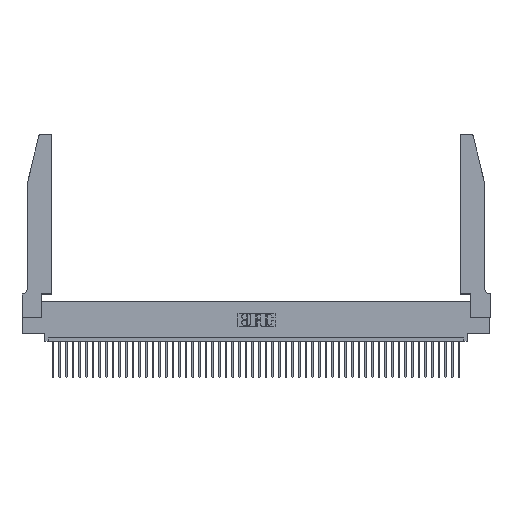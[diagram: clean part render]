
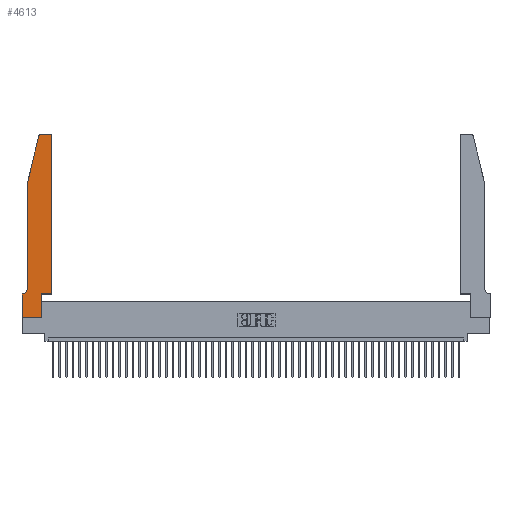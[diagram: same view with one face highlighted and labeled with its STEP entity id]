
A CAD part, top view. The second image highlights one B-rep face of the part: STEP entity #4613.
In plain terms, the highlighted planar face has unit normal (0, 0, 1).
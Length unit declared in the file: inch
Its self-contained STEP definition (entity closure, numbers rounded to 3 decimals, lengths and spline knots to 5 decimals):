
#395 = VERTEX_POINT ( 'NONE', #43126 ) ;
#557 = ORIENTED_EDGE ( 'NONE', *, *, #23836, .T. ) ;
#983 = DIRECTION ( 'NONE',  ( 0., -1., 0. ) ) ;
#1097 = CARTESIAN_POINT ( 'NONE',  ( 0.0755, 0.42, 0.37 ) ) ;
#1267 = CARTESIAN_POINT ( 'NONE',  ( 0.284, 2.72, 0.37 ) ) ;
#1682 = ORIENTED_EDGE ( 'NONE', *, *, #11763, .T. ) ;
#2705 = LINE ( 'NONE', #34800, #46370 ) ;
#3208 = CARTESIAN_POINT ( 'NONE',  ( 0.0755, 2., 0.37 ) ) ;
#3224 = ORIENTED_EDGE ( 'NONE', *, *, #18024, .T. ) ;
#3240 = VERTEX_POINT ( 'NONE', #15658 ) ;
#3483 = CIRCLE ( 'NONE', #43218, 0.03 ) ;
#4543 = LINE ( 'NONE', #46883, #14045 ) ;
#4613 = ADVANCED_FACE ( 'NONE', ( #15782 ), #11750, .T. ) ;
#5359 = VERTEX_POINT ( 'NONE', #21360 ) ;
#5878 = DIRECTION ( 'NONE',  ( -0.239, -0.971, 0. ) ) ;
#5913 = CARTESIAN_POINT ( 'NONE',  ( 0., 0., 0.37 ) ) ;
#6184 = ORIENTED_EDGE ( 'NONE', *, *, #33847, .T. ) ;
#8842 = DIRECTION ( 'NONE',  ( 0., 1., 0. ) ) ;
#9251 = VERTEX_POINT ( 'NONE', #22373 ) ;
#9542 = VECTOR ( 'NONE', #29559, 39.37008 ) ;
#10167 = CARTESIAN_POINT ( 'NONE',  ( 0.0755, 2., 0.37 ) ) ;
#10776 = LINE ( 'NONE', #3208, #9542 ) ;
#11305 = ORIENTED_EDGE ( 'NONE', *, *, #46150, .T. ) ;
#11508 = VERTEX_POINT ( 'NONE', #1097 ) ;
#11750 = PLANE ( 'NONE',  #26635 ) ;
#11763 = EDGE_CURVE ( 'NONE', #17399, #24518, #3483, .T. ) ;
#12138 = ORIENTED_EDGE ( 'NONE', *, *, #13380, .T. ) ;
#12167 = DIRECTION ( 'NONE',  ( -1., 0., 0. ) ) ;
#12723 = VECTOR ( 'NONE', #5878, 39.37008 ) ;
#13380 = EDGE_CURVE ( 'NONE', #32397, #20849, #27481, .T. ) ;
#14045 = VECTOR ( 'NONE', #28001, 39.37008 ) ;
#15224 = VECTOR ( 'NONE', #983, 39.37008 ) ;
#15658 = CARTESIAN_POINT ( 'NONE',  ( 0.2865, 0.35, 0.37 ) ) ;
#15782 = FACE_OUTER_BOUND ( 'NONE', #29788, .T. ) ;
#15824 = ORIENTED_EDGE ( 'NONE', *, *, #44892, .T. ) ;
#15880 = EDGE_CURVE ( 'NONE', #45761, #5359, #39100, .T. ) ;
#15963 = ORIENTED_EDGE ( 'NONE', *, *, #36698, .T. ) ;
#17399 = VERTEX_POINT ( 'NONE', #23423 ) ;
#17493 = EDGE_CURVE ( 'NONE', #3240, #395, #4543, .T. ) ;
#17901 = ORIENTED_EDGE ( 'NONE', *, *, #27004, .T. ) ;
#18024 = EDGE_CURVE ( 'NONE', #11508, #27484, #38205, .T. ) ;
#19718 = DIRECTION ( 'NONE',  ( 1., 0., 0. ) ) ;
#20698 = CARTESIAN_POINT ( 'NONE',  ( 0.0055, 0.35, 0.37 ) ) ;
#20849 = VERTEX_POINT ( 'NONE', #28922 ) ;
#21014 = EDGE_CURVE ( 'NONE', #20849, #11508, #10776, .T. ) ;
#21280 = DIRECTION ( 'NONE',  ( 1., 0., 0. ) ) ;
#21360 = CARTESIAN_POINT ( 'NONE',  ( 0.2865, 0., 0.37 ) ) ;
#21470 = VECTOR ( 'NONE', #47261, 39.37008 ) ;
#22373 = CARTESIAN_POINT ( 'NONE',  ( 0.284, 2.75, 0.37 ) ) ;
#22626 = LINE ( 'NONE', #43617, #21470 ) ;
#23179 = DIRECTION ( 'NONE',  ( 0., 0., 1. ) ) ;
#23423 = CARTESIAN_POINT ( 'NONE',  ( 0.4505, 2.72, 0.37 ) ) ;
#23836 = EDGE_CURVE ( 'NONE', #9251, #32397, #24278, .T. ) ;
#24278 = CIRCLE ( 'NONE', #26773, 0.03 ) ;
#24518 = VERTEX_POINT ( 'NONE', #27552 ) ;
#25367 = DIRECTION ( 'NONE',  ( 1., 0., 0. ) ) ;
#26635 = AXIS2_PLACEMENT_3D ( 'NONE', #27994, #40625, #19718 ) ;
#26773 = AXIS2_PLACEMENT_3D ( 'NONE', #1267, #23179, #27298 ) ;
#26929 = LINE ( 'NONE', #46211, #15224 ) ;
#27004 = EDGE_CURVE ( 'NONE', #33892, #45761, #26929, .T. ) ;
#27298 = DIRECTION ( 'NONE',  ( 1., 0., 0. ) ) ;
#27481 = LINE ( 'NONE', #10167, #12723 ) ;
#27484 = VERTEX_POINT ( 'NONE', #20698 ) ;
#27552 = CARTESIAN_POINT ( 'NONE',  ( 0.4205, 2.75, 0.37 ) ) ;
#27819 = DIRECTION ( 'NONE',  ( -1., 0., 0. ) ) ;
#27994 = CARTESIAN_POINT ( 'NONE',  ( 0., 0.35, 0.37 ) ) ;
#28001 = DIRECTION ( 'NONE',  ( 1., 0., 0. ) ) ;
#28160 = DIRECTION ( 'NONE',  ( 0., 0., -1. ) ) ;
#28922 = CARTESIAN_POINT ( 'NONE',  ( 0.0755, 2., 0.37 ) ) ;
#29034 = VECTOR ( 'NONE', #21280, 39.37008 ) ;
#29559 = DIRECTION ( 'NONE',  ( 0., -1., 0. ) ) ;
#29788 = EDGE_LOOP ( 'NONE', ( #6184, #557, #12138, #35660, #3224, #11305, #17901, #42258, #15963, #38117, #15824, #1682 ) ) ;
#31675 = LINE ( 'NONE', #34939, #42320 ) ;
#32397 = VERTEX_POINT ( 'NONE', #35974 ) ;
#33847 = EDGE_CURVE ( 'NONE', #24518, #9251, #31675, .T. ) ;
#33892 = VERTEX_POINT ( 'NONE', #38326 ) ;
#34800 = CARTESIAN_POINT ( 'NONE',  ( 0.2865, 0.35, 0.37 ) ) ;
#34939 = CARTESIAN_POINT ( 'NONE',  ( 0.2605, 2.75, 0.37 ) ) ;
#35604 = CARTESIAN_POINT ( 'NONE',  ( 0.0055, 0.42, 0.37 ) ) ;
#35660 = ORIENTED_EDGE ( 'NONE', *, *, #21014, .T. ) ;
#35974 = CARTESIAN_POINT ( 'NONE',  ( 0.25487, 2.72718, 0.37 ) ) ;
#36698 = EDGE_CURVE ( 'NONE', #5359, #3240, #2705, .T. ) ;
#36958 = CARTESIAN_POINT ( 'NONE',  ( 0.4205, 2.72, 0.37 ) ) ;
#37273 = CARTESIAN_POINT ( 'NONE',  ( 0., 0., 0.37 ) ) ;
#38117 = ORIENTED_EDGE ( 'NONE', *, *, #17493, .T. ) ;
#38205 = CIRCLE ( 'NONE', #43784, 0.07 ) ;
#38326 = CARTESIAN_POINT ( 'NONE',  ( 0., 0.35, 0.37 ) ) ;
#39100 = LINE ( 'NONE', #5913, #29034 ) ;
#40625 = DIRECTION ( 'NONE',  ( 0., 0., 1. ) ) ;
#42242 = VECTOR ( 'NONE', #47208, 39.37008 ) ;
#42258 = ORIENTED_EDGE ( 'NONE', *, *, #15880, .T. ) ;
#42320 = VECTOR ( 'NONE', #12167, 39.37008 ) ;
#43126 = CARTESIAN_POINT ( 'NONE',  ( 0.4505, 0.35, 0.37 ) ) ;
#43218 = AXIS2_PLACEMENT_3D ( 'NONE', #36958, #48021, #25367 ) ;
#43428 = LINE ( 'NONE', #45111, #42242 ) ;
#43617 = CARTESIAN_POINT ( 'NONE',  ( 0.0755, 0.35, 0.37 ) ) ;
#43784 = AXIS2_PLACEMENT_3D ( 'NONE', #35604, #28160, #27819 ) ;
#44892 = EDGE_CURVE ( 'NONE', #395, #17399, #43428, .T. ) ;
#45111 = CARTESIAN_POINT ( 'NONE',  ( 0.4505, 0.35, 0.37 ) ) ;
#45761 = VERTEX_POINT ( 'NONE', #37273 ) ;
#46150 = EDGE_CURVE ( 'NONE', #27484, #33892, #22626, .T. ) ;
#46211 = CARTESIAN_POINT ( 'NONE',  ( 0., 0., 0.37 ) ) ;
#46370 = VECTOR ( 'NONE', #8842, 39.37008 ) ;
#46883 = CARTESIAN_POINT ( 'NONE',  ( 0.4505, 0.35, 0.37 ) ) ;
#47208 = DIRECTION ( 'NONE',  ( 0., 1., 0. ) ) ;
#47261 = DIRECTION ( 'NONE',  ( -1., 0., 0. ) ) ;
#48021 = DIRECTION ( 'NONE',  ( 0., 0., 1. ) ) ;
